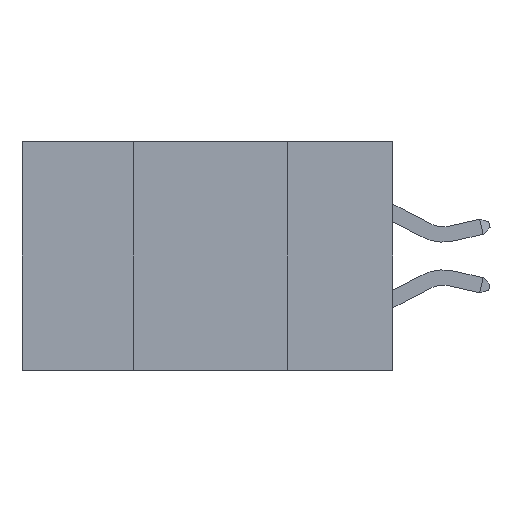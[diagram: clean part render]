
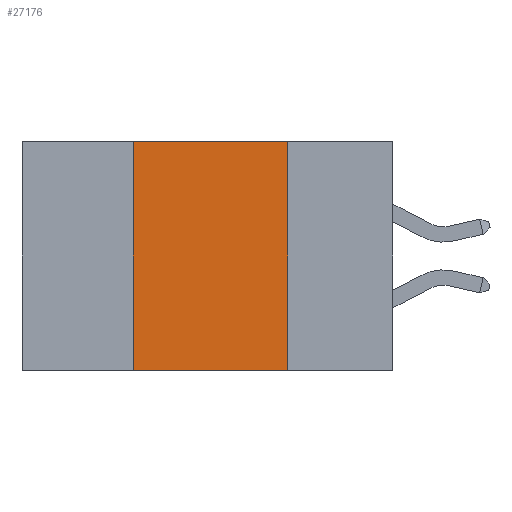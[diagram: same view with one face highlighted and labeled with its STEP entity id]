
A CAD part, left-side view. The second image highlights one B-rep face of the part: STEP entity #27176.
In plain terms, the highlighted planar face has unit normal (-1, 0, 0).
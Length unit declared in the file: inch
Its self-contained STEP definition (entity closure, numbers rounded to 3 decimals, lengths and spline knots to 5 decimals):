
#356 = VECTOR ( 'NONE', #10654, 39.37008 ) ;
#1019 = FACE_OUTER_BOUND ( 'NONE', #14903, .T. ) ;
#1365 = DIRECTION ( 'NONE',  ( 1., 0., 0. ) ) ;
#2065 = VERTEX_POINT ( 'NONE', #19622 ) ;
#3472 = ORIENTED_EDGE ( 'NONE', *, *, #26750, .F. ) ;
#4004 = DIRECTION ( 'NONE',  ( 0., 0., 1. ) ) ;
#4111 = LINE ( 'NONE', #5876, #14782 ) ;
#4158 = CARTESIAN_POINT ( 'NONE',  ( 0., 0.42, 0. ) ) ;
#4507 = CARTESIAN_POINT ( 'NONE',  ( 0., 0.17, 0. ) ) ;
#5876 = CARTESIAN_POINT ( 'NONE',  ( 0., 0.42, 0. ) ) ;
#5942 = CARTESIAN_POINT ( 'NONE',  ( 0., 0.6, 0. ) ) ;
#5945 = EDGE_CURVE ( 'NONE', #12811, #26753, #4111, .T. ) ;
#5972 = ORIENTED_EDGE ( 'NONE', *, *, #5945, .F. ) ;
#8335 = AXIS2_PLACEMENT_3D ( 'NONE', #12035, #1365, #12324 ) ;
#9472 = EDGE_CURVE ( 'NONE', #12811, #2065, #11408, .T. ) ;
#10654 = DIRECTION ( 'NONE',  ( 0., 0., -1. ) ) ;
#11408 = LINE ( 'NONE', #20682, #25732 ) ;
#11721 = LINE ( 'NONE', #5942, #20030 ) ;
#12035 = CARTESIAN_POINT ( 'NONE',  ( 0., 0.6, 0. ) ) ;
#12324 = DIRECTION ( 'NONE',  ( 0., 0., -1. ) ) ;
#12811 = VERTEX_POINT ( 'NONE', #16284 ) ;
#14385 = DIRECTION ( 'NONE',  ( 0., -1., 0. ) ) ;
#14782 = VECTOR ( 'NONE', #4004, 39.37008 ) ;
#14903 = EDGE_LOOP ( 'NONE', ( #3472, #22362, #5972, #23489 ) ) ;
#15427 = EDGE_CURVE ( 'NONE', #26753, #24031, #11721, .T. ) ;
#16284 = CARTESIAN_POINT ( 'NONE',  ( 0., 0.42, -0.37 ) ) ;
#18444 = PLANE ( 'NONE',  #8335 ) ;
#19622 = CARTESIAN_POINT ( 'NONE',  ( 0., 0.17, -0.37 ) ) ;
#20030 = VECTOR ( 'NONE', #23340, 39.37008 ) ;
#20682 = CARTESIAN_POINT ( 'NONE',  ( 0., 0.6, -0.37 ) ) ;
#22362 = ORIENTED_EDGE ( 'NONE', *, *, #15427, .F. ) ;
#23340 = DIRECTION ( 'NONE',  ( 0., -1., 0. ) ) ;
#23489 = ORIENTED_EDGE ( 'NONE', *, *, #9472, .T. ) ;
#24031 = VERTEX_POINT ( 'NONE', #27040 ) ;
#25094 = LINE ( 'NONE', #4507, #356 ) ;
#25732 = VECTOR ( 'NONE', #14385, 39.37008 ) ;
#26750 = EDGE_CURVE ( 'NONE', #24031, #2065, #25094, .T. ) ;
#26753 = VERTEX_POINT ( 'NONE', #4158 ) ;
#27040 = CARTESIAN_POINT ( 'NONE',  ( 0., 0.17, 0. ) ) ;
#27176 = ADVANCED_FACE ( 'NONE', ( #1019 ), #18444, .F. ) ;
